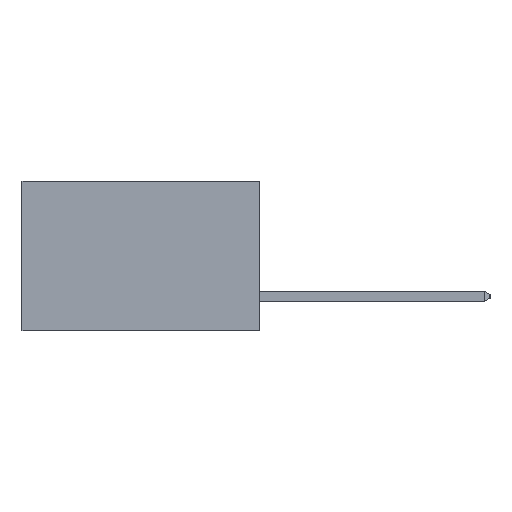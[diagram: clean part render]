
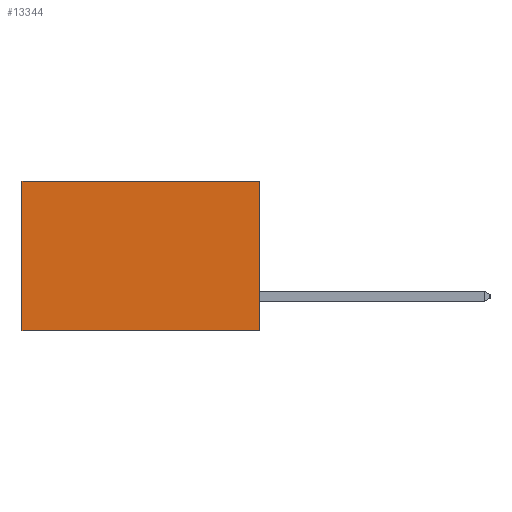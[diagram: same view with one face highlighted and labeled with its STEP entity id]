
A CAD part, left-side view. The second image highlights one B-rep face of the part: STEP entity #13344.
In plain terms, the highlighted planar face has unit normal (-1, 0, 0).
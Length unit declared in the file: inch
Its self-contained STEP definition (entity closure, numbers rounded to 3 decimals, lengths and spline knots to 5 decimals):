
#484 = AXIS2_PLACEMENT_3D ( 'NONE', #10663, #3039, #11891 ) ;
#1019 = EDGE_CURVE ( 'NONE', #7141, #13800, #14423, .T. ) ;
#1144 = VECTOR ( 'NONE', #11456, 39.37008 ) ;
#1453 = CARTESIAN_POINT ( 'NONE',  ( 0.277, 0., -0.37 ) ) ;
#1566 = VECTOR ( 'NONE', #6592, 39.37008 ) ;
#1570 = EDGE_CURVE ( 'NONE', #11966, #7141, #11266, .T. ) ;
#1741 = PLANE ( 'NONE',  #484 ) ;
#2717 = VECTOR ( 'NONE', #13218, 39.37008 ) ;
#3039 = DIRECTION ( 'NONE',  ( 1., 0., 0. ) ) ;
#5882 = CARTESIAN_POINT ( 'NONE',  ( 0.277, 0.59, -0.37 ) ) ;
#6592 = DIRECTION ( 'NONE',  ( 0., 1., 0. ) ) ;
#6830 = CARTESIAN_POINT ( 'NONE',  ( 0.277, 0., -0.37 ) ) ;
#7141 = VERTEX_POINT ( 'NONE', #1453 ) ;
#7165 = CARTESIAN_POINT ( 'NONE',  ( 0.277, 0.59, 0. ) ) ;
#7399 = LINE ( 'NONE', #5882, #10378 ) ;
#7426 = ORIENTED_EDGE ( 'NONE', *, *, #1570, .F. ) ;
#7825 = ORIENTED_EDGE ( 'NONE', *, *, #15818, .T. ) ;
#8957 = EDGE_LOOP ( 'NONE', ( #9633, #15894, #7426, #7825 ) ) ;
#9483 = FACE_OUTER_BOUND ( 'NONE', #8957, .T. ) ;
#9633 = ORIENTED_EDGE ( 'NONE', *, *, #9786, .T. ) ;
#9786 = EDGE_CURVE ( 'NONE', #14145, #13800, #7399, .T. ) ;
#10378 = VECTOR ( 'NONE', #15554, 39.37008 ) ;
#10663 = CARTESIAN_POINT ( 'NONE',  ( 0.277, 0., -0.37 ) ) ;
#11266 = LINE ( 'NONE', #11536, #1144 ) ;
#11456 = DIRECTION ( 'NONE',  ( 0., 0., -1. ) ) ;
#11536 = CARTESIAN_POINT ( 'NONE',  ( 0.277, 0., -0.37 ) ) ;
#11891 = DIRECTION ( 'NONE',  ( 0., 0., -1. ) ) ;
#11966 = VERTEX_POINT ( 'NONE', #13986 ) ;
#12052 = CARTESIAN_POINT ( 'NONE',  ( 0.277, 0., 0. ) ) ;
#13218 = DIRECTION ( 'NONE',  ( 0., 1., 0. ) ) ;
#13344 = ADVANCED_FACE ( 'NONE', ( #9483 ), #1741, .F. ) ;
#13800 = VERTEX_POINT ( 'NONE', #15910 ) ;
#13986 = CARTESIAN_POINT ( 'NONE',  ( 0.277, 0., 0. ) ) ;
#14145 = VERTEX_POINT ( 'NONE', #7165 ) ;
#14423 = LINE ( 'NONE', #6830, #1566 ) ;
#15554 = DIRECTION ( 'NONE',  ( 0., 0., -1. ) ) ;
#15789 = LINE ( 'NONE', #12052, #2717 ) ;
#15818 = EDGE_CURVE ( 'NONE', #11966, #14145, #15789, .T. ) ;
#15894 = ORIENTED_EDGE ( 'NONE', *, *, #1019, .F. ) ;
#15910 = CARTESIAN_POINT ( 'NONE',  ( 0.277, 0.59, -0.37 ) ) ;
